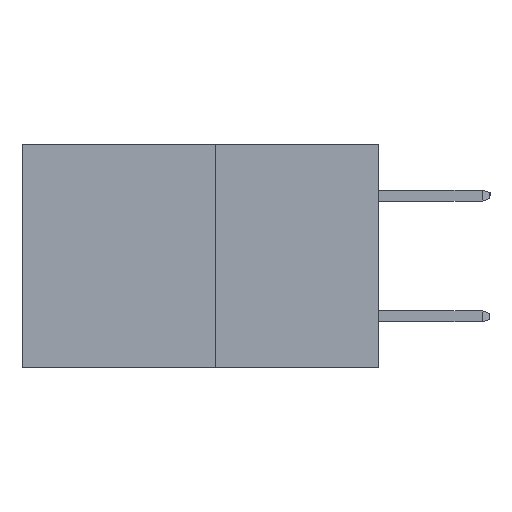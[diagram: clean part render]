
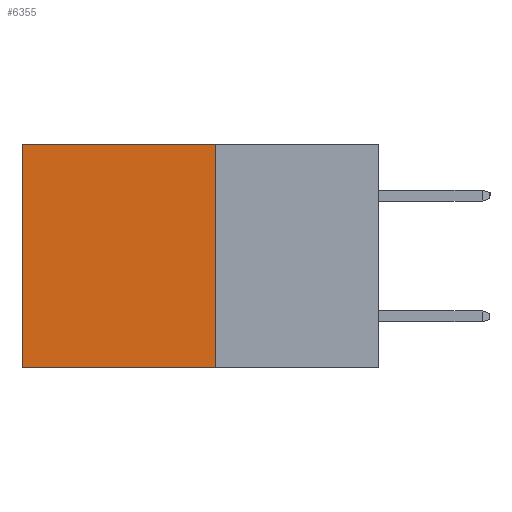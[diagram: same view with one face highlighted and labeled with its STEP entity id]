
A CAD part, left-side view. The second image highlights one B-rep face of the part: STEP entity #6355.
In plain terms, the highlighted planar face has unit normal (-1, 0, 0).
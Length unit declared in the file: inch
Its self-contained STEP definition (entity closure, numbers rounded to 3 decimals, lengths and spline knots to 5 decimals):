
#9 = DIRECTION ( 'NONE',  ( 0., 0., -1. ) ) ;
#782 = CARTESIAN_POINT ( 'NONE',  ( 0.277, 0.59, -0.37 ) ) ;
#944 = CARTESIAN_POINT ( 'NONE',  ( 0.277, 0.59, -0.37 ) ) ;
#979 = VECTOR ( 'NONE', #6088, 39.37008 ) ;
#1148 = PLANE ( 'NONE',  #4014 ) ;
#1236 = VERTEX_POINT ( 'NONE', #8148 ) ;
#1357 = ORIENTED_EDGE ( 'NONE', *, *, #6976, .T. ) ;
#2244 = VERTEX_POINT ( 'NONE', #6147 ) ;
#2540 = EDGE_CURVE ( 'NONE', #2244, #10055, #6354, .T. ) ;
#2892 = DIRECTION ( 'NONE',  ( 0., 0., -1. ) ) ;
#3683 = ORIENTED_EDGE ( 'NONE', *, *, #6176, .F. ) ;
#4014 = AXIS2_PLACEMENT_3D ( 'NONE', #7061, #7880, #2892 ) ;
#4146 = VERTEX_POINT ( 'NONE', #782 ) ;
#5149 = FACE_OUTER_BOUND ( 'NONE', #5242, .T. ) ;
#5206 = EDGE_CURVE ( 'NONE', #1236, #4146, #8574, .T. ) ;
#5219 = ORIENTED_EDGE ( 'NONE', *, *, #2540, .T. ) ;
#5242 = EDGE_LOOP ( 'NONE', ( #1357, #6572, #3683, #5219 ) ) ;
#6088 = DIRECTION ( 'NONE',  ( 0., 0., -1. ) ) ;
#6115 = DIRECTION ( 'NONE',  ( 0., 1., 0. ) ) ;
#6147 = CARTESIAN_POINT ( 'NONE',  ( 0.277, 0.27, 0. ) ) ;
#6176 = EDGE_CURVE ( 'NONE', #2244, #1236, #7461, .T. ) ;
#6354 = LINE ( 'NONE', #9419, #10279 ) ;
#6355 = ADVANCED_FACE ( 'NONE', ( #5149 ), #1148, .F. ) ;
#6453 = DIRECTION ( 'NONE',  ( 0., 1., 0. ) ) ;
#6572 = ORIENTED_EDGE ( 'NONE', *, *, #5206, .F. ) ;
#6976 = EDGE_CURVE ( 'NONE', #10055, #4146, #10240, .T. ) ;
#7061 = CARTESIAN_POINT ( 'NONE',  ( 0.277, 0.27, -0.37 ) ) ;
#7213 = VECTOR ( 'NONE', #9, 39.37008 ) ;
#7295 = CARTESIAN_POINT ( 'NONE',  ( 0.277, 0.27, -0.37 ) ) ;
#7461 = LINE ( 'NONE', #9979, #7213 ) ;
#7588 = CARTESIAN_POINT ( 'NONE',  ( 0.277, 0.59, 0. ) ) ;
#7880 = DIRECTION ( 'NONE',  ( 1., 0., 0. ) ) ;
#8148 = CARTESIAN_POINT ( 'NONE',  ( 0.277, 0.27, -0.37 ) ) ;
#8574 = LINE ( 'NONE', #7295, #8815 ) ;
#8815 = VECTOR ( 'NONE', #6453, 39.37008 ) ;
#9419 = CARTESIAN_POINT ( 'NONE',  ( 0.277, 0.27, 0. ) ) ;
#9979 = CARTESIAN_POINT ( 'NONE',  ( 0.277, 0.27, -0.37 ) ) ;
#10055 = VERTEX_POINT ( 'NONE', #7588 ) ;
#10240 = LINE ( 'NONE', #944, #979 ) ;
#10279 = VECTOR ( 'NONE', #6115, 39.37008 ) ;
